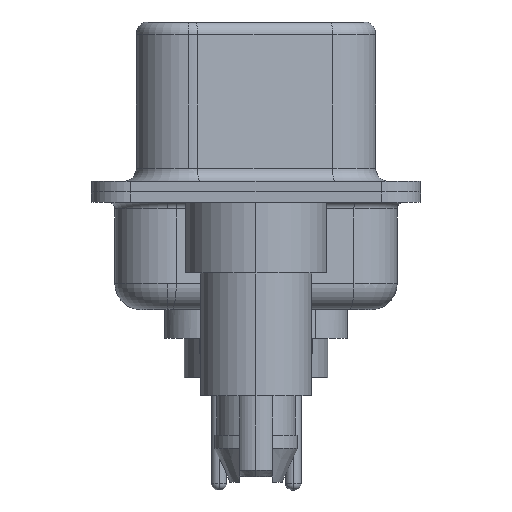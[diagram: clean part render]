
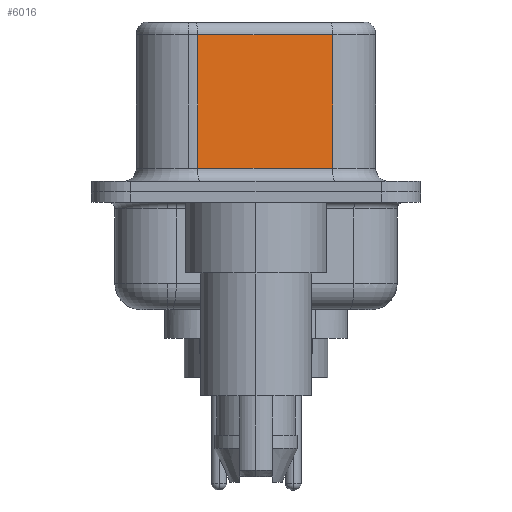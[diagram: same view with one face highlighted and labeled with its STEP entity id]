
A CAD part, left-side view. The second image highlights one B-rep face of the part: STEP entity #6016.
In plain terms, the highlighted planar face has unit normal (-0.985, -0.174, 0).
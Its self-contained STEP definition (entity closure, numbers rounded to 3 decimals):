
#70 = EDGE_CURVE ( 'NONE', #10449, #11577, #5211, .T. ) ;
#268 = ORIENTED_EDGE ( 'NONE', *, *, #14125, .F. ) ;
#402 = LINE ( 'NONE', #15596, #18074 ) ;
#1783 = LINE ( 'NONE', #5255, #2336 ) ;
#2336 = VECTOR ( 'NONE', #10794, 1000. ) ;
#3785 = VERTEX_POINT ( 'NONE', #13930 ) ;
#4472 = EDGE_CURVE ( 'NONE', #3785, #21314, #1783, .T. ) ;
#4969 = ORIENTED_EDGE ( 'NONE', *, *, #70, .T. ) ;
#5211 = LINE ( 'NONE', #10552, #8179 ) ;
#5255 = CARTESIAN_POINT ( 'NONE',  ( 4.565, -2.927, 0.9 ) ) ;
#5325 = DIRECTION ( 'NONE',  ( 0., 0., -1. ) ) ;
#5861 = FACE_OUTER_BOUND ( 'NONE', #20974, .T. ) ;
#5949 = DIRECTION ( 'NONE',  ( -0.174, 0.985, 0. ) ) ;
#6012 = DIRECTION ( 'NONE',  ( 0., 0., -1. ) ) ;
#6016 = ADVANCED_FACE ( 'NONE', ( #5861 ), #19899, .F. ) ;
#6170 = DIRECTION ( 'NONE',  ( 0.985, 0.174, 0. ) ) ;
#6247 = CARTESIAN_POINT ( 'NONE',  ( 4.565, -2.927, 6.52 ) ) ;
#7688 = CARTESIAN_POINT ( 'NONE',  ( 4.565, -2.927, 0.9 ) ) ;
#8179 = VECTOR ( 'NONE', #8540, 1000. ) ;
#8540 = DIRECTION ( 'NONE',  ( -0.174, 0.985, 0. ) ) ;
#10449 = VERTEX_POINT ( 'NONE', #11298 ) ;
#10552 = CARTESIAN_POINT ( 'NONE',  ( 4.565, -2.927, 6.02 ) ) ;
#10677 = AXIS2_PLACEMENT_3D ( 'NONE', #6247, #6170, #5949 ) ;
#10794 = DIRECTION ( 'NONE',  ( 0.174, -0.985, 0. ) ) ;
#11298 = CARTESIAN_POINT ( 'NONE',  ( 4.565, -2.927, 6.02 ) ) ;
#11577 = VERTEX_POINT ( 'NONE', #12662 ) ;
#12516 = EDGE_CURVE ( 'NONE', #11577, #3785, #14490, .T. ) ;
#12662 = CARTESIAN_POINT ( 'NONE',  ( 3.655, 2.233, 6.02 ) ) ;
#12803 = ORIENTED_EDGE ( 'NONE', *, *, #12516, .T. ) ;
#13930 = CARTESIAN_POINT ( 'NONE',  ( 3.655, 2.233, 0.9 ) ) ;
#14125 = EDGE_CURVE ( 'NONE', #10449, #21314, #402, .T. ) ;
#14490 = LINE ( 'NONE', #17900, #19449 ) ;
#15596 = CARTESIAN_POINT ( 'NONE',  ( 4.565, -2.927, 6.52 ) ) ;
#17900 = CARTESIAN_POINT ( 'NONE',  ( 3.655, 2.233, 6.52 ) ) ;
#18074 = VECTOR ( 'NONE', #5325, 1000. ) ;
#19449 = VECTOR ( 'NONE', #6012, 1000. ) ;
#19899 = PLANE ( 'NONE',  #10677 ) ;
#20249 = ORIENTED_EDGE ( 'NONE', *, *, #4472, .T. ) ;
#20974 = EDGE_LOOP ( 'NONE', ( #268, #4969, #12803, #20249 ) ) ;
#21314 = VERTEX_POINT ( 'NONE', #7688 ) ;
